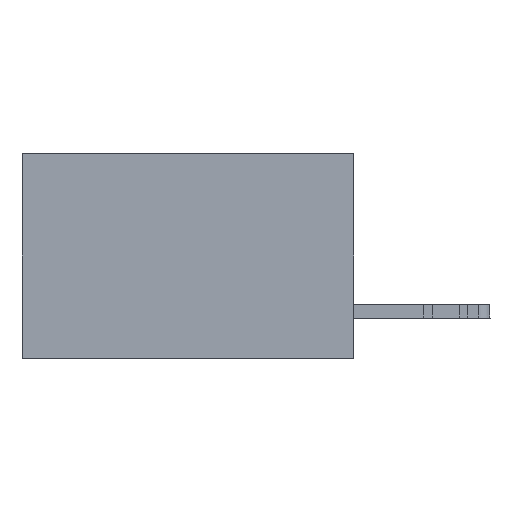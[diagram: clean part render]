
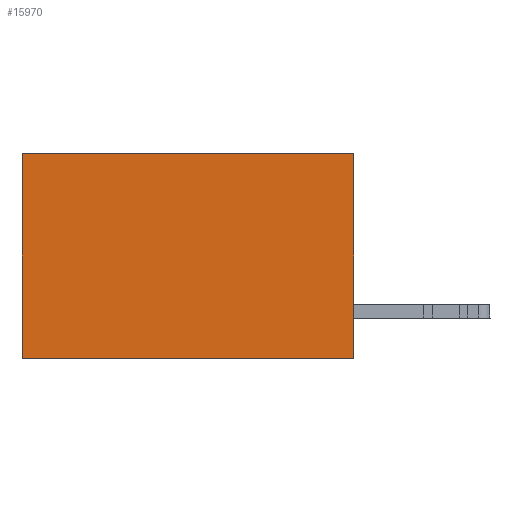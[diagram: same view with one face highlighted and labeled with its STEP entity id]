
A CAD part, left-side view. The second image highlights one B-rep face of the part: STEP entity #15970.
In plain terms, the highlighted planar face has unit normal (-1, 0, 0).
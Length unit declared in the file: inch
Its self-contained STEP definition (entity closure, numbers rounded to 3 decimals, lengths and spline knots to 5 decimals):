
#2306 = DIRECTION ( 'NONE',  ( 0., 0., -1. ) ) ;
#2318 = EDGE_LOOP ( 'NONE', ( #40030, #8805, #8554, #14378 ) ) ;
#3183 = AXIS2_PLACEMENT_3D ( 'NONE', #19527, #33377, #2306 ) ;
#3562 = LINE ( 'NONE', #17410, #25468 ) ;
#5709 = PLANE ( 'NONE',  #3183 ) ;
#6519 = VERTEX_POINT ( 'NONE', #40957 ) ;
#8554 = ORIENTED_EDGE ( 'NONE', *, *, #39339, .F. ) ;
#8571 = CARTESIAN_POINT ( 'NONE',  ( 0.2875, 0., 0. ) ) ;
#8805 = ORIENTED_EDGE ( 'NONE', *, *, #25321, .F. ) ;
#10275 = CARTESIAN_POINT ( 'NONE',  ( 0.2875, 0., -0.37 ) ) ;
#11219 = VERTEX_POINT ( 'NONE', #26101 ) ;
#11750 = LINE ( 'NONE', #25786, #12081 ) ;
#12081 = VECTOR ( 'NONE', #39871, 39.37008 ) ;
#14378 = ORIENTED_EDGE ( 'NONE', *, *, #34006, .T. ) ;
#15177 = VECTOR ( 'NONE', #22379, 39.37008 ) ;
#15970 = ADVANCED_FACE ( 'NONE', ( #22245 ), #5709, .F. ) ;
#16883 = VECTOR ( 'NONE', #41234, 39.37008 ) ;
#17410 = CARTESIAN_POINT ( 'NONE',  ( 0.2875, 0., -0.37 ) ) ;
#17774 = VERTEX_POINT ( 'NONE', #31282 ) ;
#19527 = CARTESIAN_POINT ( 'NONE',  ( 0.2875, 0., 0. ) ) ;
#22245 = FACE_OUTER_BOUND ( 'NONE', #2318, .T. ) ;
#22379 = DIRECTION ( 'NONE',  ( 0., 0., -1. ) ) ;
#24650 = DIRECTION ( 'NONE',  ( 0., 1., 0. ) ) ;
#25321 = EDGE_CURVE ( 'NONE', #34548, #17774, #3562, .T. ) ;
#25468 = VECTOR ( 'NONE', #24650, 39.37008 ) ;
#25786 = CARTESIAN_POINT ( 'NONE',  ( 0.2875, 0., 0. ) ) ;
#26101 = CARTESIAN_POINT ( 'NONE',  ( 0.2875, 0., 0. ) ) ;
#26555 = EDGE_CURVE ( 'NONE', #6519, #17774, #27392, .T. ) ;
#27392 = LINE ( 'NONE', #38264, #16883 ) ;
#31282 = CARTESIAN_POINT ( 'NONE',  ( 0.2875, 0.6, -0.37 ) ) ;
#33377 = DIRECTION ( 'NONE',  ( 1., 0., 0. ) ) ;
#34006 = EDGE_CURVE ( 'NONE', #11219, #6519, #11750, .T. ) ;
#34548 = VERTEX_POINT ( 'NONE', #10275 ) ;
#36239 = LINE ( 'NONE', #8571, #15177 ) ;
#38264 = CARTESIAN_POINT ( 'NONE',  ( 0.2875, 0.6, 0. ) ) ;
#39339 = EDGE_CURVE ( 'NONE', #11219, #34548, #36239, .T. ) ;
#39871 = DIRECTION ( 'NONE',  ( 0., 1., 0. ) ) ;
#40030 = ORIENTED_EDGE ( 'NONE', *, *, #26555, .T. ) ;
#40957 = CARTESIAN_POINT ( 'NONE',  ( 0.2875, 0.6, 0. ) ) ;
#41234 = DIRECTION ( 'NONE',  ( 0., 0., -1. ) ) ;
